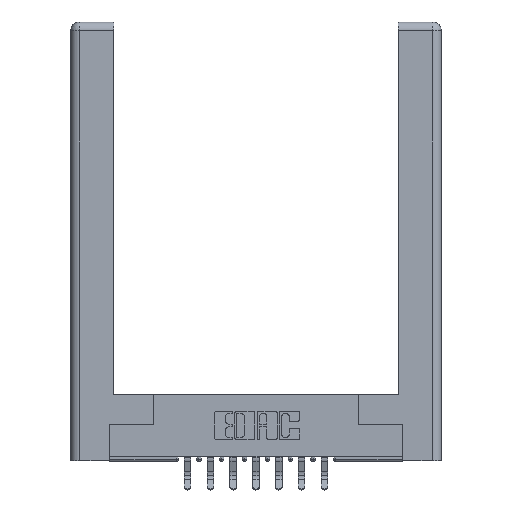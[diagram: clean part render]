
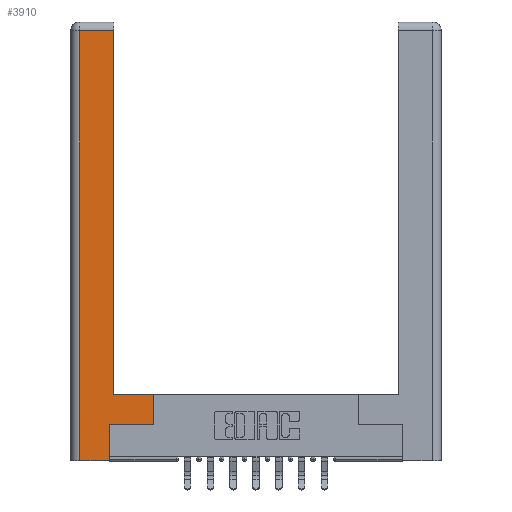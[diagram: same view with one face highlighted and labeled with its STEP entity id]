
A CAD part, top view. The second image highlights one B-rep face of the part: STEP entity #3910.
In plain terms, the highlighted planar face has unit normal (0, 0, 1).
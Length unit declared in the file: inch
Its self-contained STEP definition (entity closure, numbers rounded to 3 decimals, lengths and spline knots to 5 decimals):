
#298 = VECTOR ( 'NONE', #3738, 39.37008 ) ;
#435 = CARTESIAN_POINT ( 'NONE',  ( 0.0615, 2.94, 0. ) ) ;
#636 = CARTESIAN_POINT ( 'NONE',  ( 0.265, 0., 0. ) ) ;
#939 = DIRECTION ( 'NONE',  ( 0., -1., 0. ) ) ;
#957 = DIRECTION ( 'NONE',  ( -1., 0., 0. ) ) ;
#1595 = CARTESIAN_POINT ( 'NONE',  ( 0.565, 0.245, 0. ) ) ;
#1610 = DIRECTION ( 'NONE',  ( 0., 1., 0. ) ) ;
#1661 = LINE ( 'NONE', #14343, #3605 ) ;
#1888 = EDGE_CURVE ( 'NONE', #3031, #3536, #14554, .T. ) ;
#2140 = DIRECTION ( 'NONE',  ( 1., 0., 0. ) ) ;
#2219 = LINE ( 'NONE', #3848, #10586 ) ;
#2241 = ORIENTED_EDGE ( 'NONE', *, *, #3859, .T. ) ;
#2462 = EDGE_CURVE ( 'NONE', #11536, #8008, #6313, .T. ) ;
#2517 = VECTOR ( 'NONE', #6327, 39.37008 ) ;
#2768 = EDGE_CURVE ( 'NONE', #7959, #11536, #14340, .T. ) ;
#2889 = EDGE_CURVE ( 'NONE', #8552, #3031, #4003, .T. ) ;
#3031 = VERTEX_POINT ( 'NONE', #1595 ) ;
#3245 = PLANE ( 'NONE',  #10183 ) ;
#3288 = CARTESIAN_POINT ( 'NONE',  ( 0.565, 0.245, 0. ) ) ;
#3331 = CARTESIAN_POINT ( 'NONE',  ( 0.295, 2.94, 0. ) ) ;
#3536 = VERTEX_POINT ( 'NONE', #3691 ) ;
#3605 = VECTOR ( 'NONE', #1610, 39.37008 ) ;
#3679 = EDGE_CURVE ( 'NONE', #8535, #8552, #1661, .T. ) ;
#3691 = CARTESIAN_POINT ( 'NONE',  ( 0.565, 0.45, 0. ) ) ;
#3738 = DIRECTION ( 'NONE',  ( -1., 0., 0. ) ) ;
#3848 = CARTESIAN_POINT ( 'NONE',  ( 0.265, 0., 0. ) ) ;
#3859 = EDGE_CURVE ( 'NONE', #3536, #5237, #13065, .T. ) ;
#3910 = ADVANCED_FACE ( 'NONE', ( #5004 ), #3245, .F. ) ;
#4003 = LINE ( 'NONE', #3288, #4695 ) ;
#4245 = CARTESIAN_POINT ( 'NONE',  ( 0.0615, 2.94, 0. ) ) ;
#4307 = ORIENTED_EDGE ( 'NONE', *, *, #2889, .T. ) ;
#4400 = DIRECTION ( 'NONE',  ( 0., 0., -1. ) ) ;
#4695 = VECTOR ( 'NONE', #2140, 39.37008 ) ;
#5004 = FACE_OUTER_BOUND ( 'NONE', #11856, .T. ) ;
#5180 = CARTESIAN_POINT ( 'NONE',  ( 0.295, 3., 0. ) ) ;
#5237 = VERTEX_POINT ( 'NONE', #7840 ) ;
#5497 = CARTESIAN_POINT ( 'NONE',  ( 0., 0., 0. ) ) ;
#5787 = DIRECTION ( 'NONE',  ( -1., 0., 0. ) ) ;
#5966 = VECTOR ( 'NONE', #7903, 39.37008 ) ;
#5975 = ORIENTED_EDGE ( 'NONE', *, *, #1888, .T. ) ;
#6313 = LINE ( 'NONE', #12421, #11880 ) ;
#6327 = DIRECTION ( 'NONE',  ( 0., 1., 0. ) ) ;
#6738 = CARTESIAN_POINT ( 'NONE',  ( 0.0615, 0., 0. ) ) ;
#7803 = CARTESIAN_POINT ( 'NONE',  ( 0.295, 0.45, 0. ) ) ;
#7840 = CARTESIAN_POINT ( 'NONE',  ( 0.295, 0.45, 0. ) ) ;
#7903 = DIRECTION ( 'NONE',  ( 0., 1., 0. ) ) ;
#7959 = VERTEX_POINT ( 'NONE', #3331 ) ;
#8008 = VERTEX_POINT ( 'NONE', #6738 ) ;
#8535 = VERTEX_POINT ( 'NONE', #636 ) ;
#8548 = ORIENTED_EDGE ( 'NONE', *, *, #10264, .T. ) ;
#8552 = VERTEX_POINT ( 'NONE', #11989 ) ;
#8579 = DIRECTION ( 'NONE',  ( 1., 0., 0. ) ) ;
#9456 = LINE ( 'NONE', #5180, #2517 ) ;
#10183 = AXIS2_PLACEMENT_3D ( 'NONE', #5497, #4400, #5787 ) ;
#10264 = EDGE_CURVE ( 'NONE', #5237, #7959, #9456, .T. ) ;
#10586 = VECTOR ( 'NONE', #8579, 39.37008 ) ;
#11536 = VERTEX_POINT ( 'NONE', #4245 ) ;
#11856 = EDGE_LOOP ( 'NONE', ( #8548, #12045, #13423, #13829, #13771, #4307, #5975, #2241 ) ) ;
#11880 = VECTOR ( 'NONE', #939, 39.37008 ) ;
#11989 = CARTESIAN_POINT ( 'NONE',  ( 0.265, 0.245, 0. ) ) ;
#12045 = ORIENTED_EDGE ( 'NONE', *, *, #2768, .T. ) ;
#12421 = CARTESIAN_POINT ( 'NONE',  ( 0.0615, 0., 0. ) ) ;
#13065 = LINE ( 'NONE', #7803, #14474 ) ;
#13375 = CARTESIAN_POINT ( 'NONE',  ( 0.565, 0.45, 0. ) ) ;
#13423 = ORIENTED_EDGE ( 'NONE', *, *, #2462, .T. ) ;
#13771 = ORIENTED_EDGE ( 'NONE', *, *, #3679, .T. ) ;
#13829 = ORIENTED_EDGE ( 'NONE', *, *, #14081, .T. ) ;
#14081 = EDGE_CURVE ( 'NONE', #8008, #8535, #2219, .T. ) ;
#14340 = LINE ( 'NONE', #435, #298 ) ;
#14343 = CARTESIAN_POINT ( 'NONE',  ( 0.265, 0.245, 0. ) ) ;
#14474 = VECTOR ( 'NONE', #957, 39.37008 ) ;
#14554 = LINE ( 'NONE', #13375, #5966 ) ;
